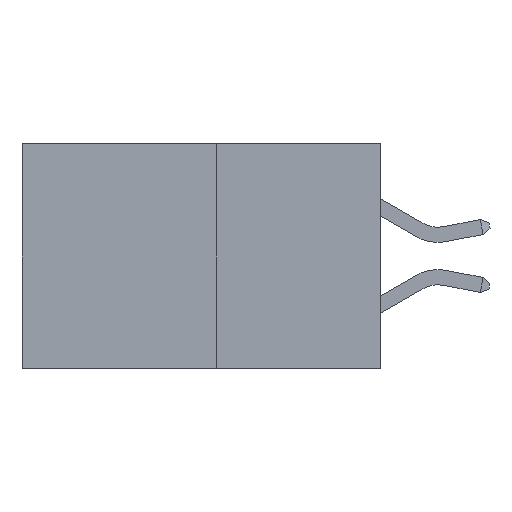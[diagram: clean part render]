
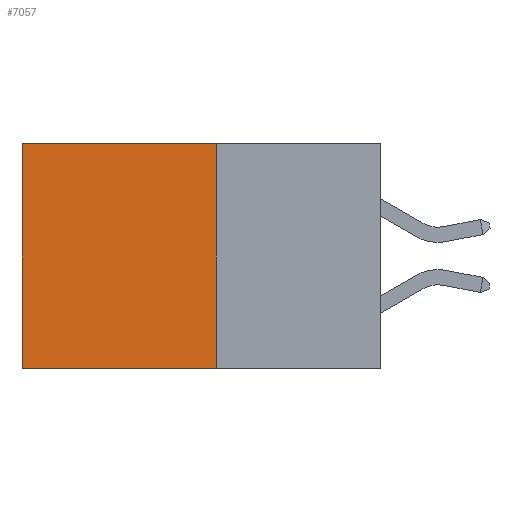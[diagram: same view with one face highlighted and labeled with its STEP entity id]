
A CAD part, left-side view. The second image highlights one B-rep face of the part: STEP entity #7057.
In plain terms, the highlighted planar face has unit normal (-1, 0, 0).
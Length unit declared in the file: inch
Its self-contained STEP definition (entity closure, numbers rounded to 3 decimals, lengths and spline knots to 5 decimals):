
#506 = VERTEX_POINT ( 'NONE', #2707 ) ;
#1200 = EDGE_CURVE ( 'NONE', #10048, #5896, #4115, .T. ) ;
#1247 = CARTESIAN_POINT ( 'NONE',  ( 0.277, 0.59, 0. ) ) ;
#1381 = ORIENTED_EDGE ( 'NONE', *, *, #5827, .T. ) ;
#1649 = ORIENTED_EDGE ( 'NONE', *, *, #5337, .F. ) ;
#1924 = VECTOR ( 'NONE', #5074, 39.37008 ) ;
#1982 = DIRECTION ( 'NONE',  ( 0., 1., 0. ) ) ;
#2160 = CARTESIAN_POINT ( 'NONE',  ( 0.277, 0.59, -0.37 ) ) ;
#2225 = CARTESIAN_POINT ( 'NONE',  ( 0.277, 0.27, -0.37 ) ) ;
#2581 = ORIENTED_EDGE ( 'NONE', *, *, #1200, .T. ) ;
#2707 = CARTESIAN_POINT ( 'NONE',  ( 0.277, 0.27, 0. ) ) ;
#2856 = DIRECTION ( 'NONE',  ( 0., 0., -1. ) ) ;
#2939 = DIRECTION ( 'NONE',  ( 0., 0., -1. ) ) ;
#3390 = VERTEX_POINT ( 'NONE', #5362 ) ;
#3495 = FACE_OUTER_BOUND ( 'NONE', #8853, .T. ) ;
#4115 = LINE ( 'NONE', #7892, #1924 ) ;
#4192 = DIRECTION ( 'NONE',  ( 0., 1., 0. ) ) ;
#4275 = VECTOR ( 'NONE', #1982, 39.37008 ) ;
#4442 = CARTESIAN_POINT ( 'NONE',  ( 0.277, 0.27, -0.37 ) ) ;
#4513 = LINE ( 'NONE', #2225, #8418 ) ;
#5074 = DIRECTION ( 'NONE',  ( 0., 0., -1. ) ) ;
#5337 = EDGE_CURVE ( 'NONE', #506, #3390, #4513, .T. ) ;
#5362 = CARTESIAN_POINT ( 'NONE',  ( 0.277, 0.27, -0.37 ) ) ;
#5827 = EDGE_CURVE ( 'NONE', #506, #10048, #6380, .T. ) ;
#5896 = VERTEX_POINT ( 'NONE', #2160 ) ;
#5926 = DIRECTION ( 'NONE',  ( 1., 0., 0. ) ) ;
#6353 = AXIS2_PLACEMENT_3D ( 'NONE', #10028, #5926, #2939 ) ;
#6380 = LINE ( 'NONE', #8525, #4275 ) ;
#6419 = VECTOR ( 'NONE', #4192, 39.37008 ) ;
#7057 = ADVANCED_FACE ( 'NONE', ( #3495 ), #9177, .F. ) ;
#7892 = CARTESIAN_POINT ( 'NONE',  ( 0.277, 0.59, -0.37 ) ) ;
#8007 = ORIENTED_EDGE ( 'NONE', *, *, #8378, .F. ) ;
#8378 = EDGE_CURVE ( 'NONE', #3390, #5896, #8446, .T. ) ;
#8418 = VECTOR ( 'NONE', #2856, 39.37008 ) ;
#8446 = LINE ( 'NONE', #4442, #6419 ) ;
#8525 = CARTESIAN_POINT ( 'NONE',  ( 0.277, 0.27, 0. ) ) ;
#8853 = EDGE_LOOP ( 'NONE', ( #2581, #8007, #1649, #1381 ) ) ;
#9177 = PLANE ( 'NONE',  #6353 ) ;
#10028 = CARTESIAN_POINT ( 'NONE',  ( 0.277, 0.27, -0.37 ) ) ;
#10048 = VERTEX_POINT ( 'NONE', #1247 ) ;
